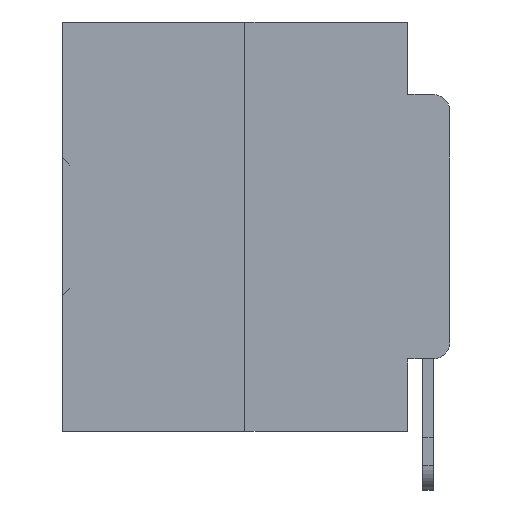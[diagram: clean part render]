
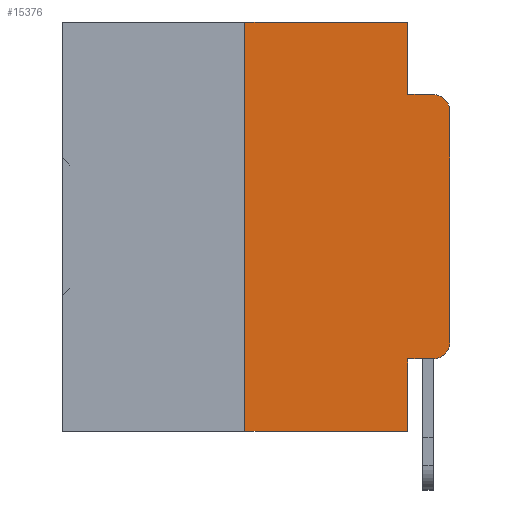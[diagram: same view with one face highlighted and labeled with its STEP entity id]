
A CAD part, left-side view. The second image highlights one B-rep face of the part: STEP entity #15376.
In plain terms, the highlighted planar face has unit normal (-1, 0, 0).
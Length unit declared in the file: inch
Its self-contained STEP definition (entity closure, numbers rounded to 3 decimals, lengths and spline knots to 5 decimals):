
#471 = CARTESIAN_POINT ( 'NONE',  ( 0., 0.02, -0.0885 ) ) ;
#874 = VECTOR ( 'NONE', #18896, 39.37008 ) ;
#1445 = VERTEX_POINT ( 'NONE', #471 ) ;
#1969 = LINE ( 'NONE', #17350, #16492 ) ;
#2561 = VECTOR ( 'NONE', #5907, 39.37008 ) ;
#3018 = DIRECTION ( 'NONE',  ( 0., 0., 1. ) ) ;
#3199 = EDGE_CURVE ( 'NONE', #34035, #13977, #10397, .T. ) ;
#3490 = LINE ( 'NONE', #34372, #25398 ) ;
#3842 = VERTEX_POINT ( 'NONE', #23069 ) ;
#4483 = EDGE_LOOP ( 'NONE', ( #11422, #12187, #13120, #13245, #14079, #14482, #14548, #14846, #14946, #15861 ) ) ;
#4899 = DIRECTION ( 'NONE',  ( -1., 0., 0. ) ) ;
#5907 = DIRECTION ( 'NONE',  ( 0., 0., -1. ) ) ;
#6653 = VERTEX_POINT ( 'NONE', #32806 ) ;
#7914 = EDGE_CURVE ( 'NONE', #28698, #6653, #32557, .T. ) ;
#8669 = PLANE ( 'NONE',  #24336 ) ;
#8960 = VECTOR ( 'NONE', #3018, 39.37008 ) ;
#9853 = CARTESIAN_POINT ( 'NONE',  ( 0., 0.051, -0.4115 ) ) ;
#10044 = EDGE_CURVE ( 'NONE', #27530, #11202, #34111, .T. ) ;
#10397 = LINE ( 'NONE', #20158, #2561 ) ;
#10764 = FACE_OUTER_BOUND ( 'NONE', #4483, .T. ) ;
#11067 = EDGE_CURVE ( 'NONE', #16762, #3842, #1969, .T. ) ;
#11202 = VERTEX_POINT ( 'NONE', #20789 ) ;
#11422 = ORIENTED_EDGE ( 'NONE', *, *, #26827, .T. ) ;
#11485 = LINE ( 'NONE', #9853, #19003 ) ;
#11572 = DIRECTION ( 'NONE',  ( 1., 0., 0. ) ) ;
#12187 = ORIENTED_EDGE ( 'NONE', *, *, #23247, .T. ) ;
#12735 = DIRECTION ( 'NONE',  ( 0., -1., 0. ) ) ;
#12960 = DIRECTION ( 'NONE',  ( 0., -1., 0. ) ) ;
#13120 = ORIENTED_EDGE ( 'NONE', *, *, #17575, .F. ) ;
#13232 = CIRCLE ( 'NONE', #33168, 0.02 ) ;
#13245 = ORIENTED_EDGE ( 'NONE', *, *, #10044, .F. ) ;
#13977 = VERTEX_POINT ( 'NONE', #35650 ) ;
#14079 = ORIENTED_EDGE ( 'NONE', *, *, #27481, .F. ) ;
#14482 = ORIENTED_EDGE ( 'NONE', *, *, #11067, .F. ) ;
#14548 = ORIENTED_EDGE ( 'NONE', *, *, #27076, .T. ) ;
#14846 = ORIENTED_EDGE ( 'NONE', *, *, #3199, .F. ) ;
#14858 = DIRECTION ( 'NONE',  ( -1., 0., 0. ) ) ;
#14946 = ORIENTED_EDGE ( 'NONE', *, *, #17477, .T. ) ;
#15376 = ADVANCED_FACE ( 'NONE', ( #10764 ), #8669, .F. ) ;
#15643 = LINE ( 'NONE', #20247, #8960 ) ;
#15861 = ORIENTED_EDGE ( 'NONE', *, *, #7914, .T. ) ;
#16492 = VECTOR ( 'NONE', #20188, 39.37008 ) ;
#16762 = VERTEX_POINT ( 'NONE', #34715 ) ;
#17074 = VECTOR ( 'NONE', #12960, 39.37008 ) ;
#17350 = CARTESIAN_POINT ( 'NONE',  ( 0., 0.25, 0. ) ) ;
#17477 = EDGE_CURVE ( 'NONE', #34035, #28698, #11485, .T. ) ;
#17575 = EDGE_CURVE ( 'NONE', #11202, #1445, #24713, .T. ) ;
#18618 = CARTESIAN_POINT ( 'NONE',  ( 0., 0.473, -0.5 ) ) ;
#18896 = DIRECTION ( 'NONE',  ( 0., -1., 0. ) ) ;
#19003 = VECTOR ( 'NONE', #12735, 39.37008 ) ;
#19226 = VECTOR ( 'NONE', #32627, 39.37008 ) ;
#20158 = CARTESIAN_POINT ( 'NONE',  ( 0., 0.051, 0. ) ) ;
#20188 = DIRECTION ( 'NONE',  ( 0., 0., 1. ) ) ;
#20247 = CARTESIAN_POINT ( 'NONE',  ( 0., 0., 0. ) ) ;
#20789 = CARTESIAN_POINT ( 'NONE',  ( 0., 0.051, -0.0885 ) ) ;
#22041 = CARTESIAN_POINT ( 'NONE',  ( 0., 0.02, -0.1085 ) ) ;
#23069 = CARTESIAN_POINT ( 'NONE',  ( 0., 0.25, 0. ) ) ;
#23247 = EDGE_CURVE ( 'NONE', #31879, #1445, #13232, .T. ) ;
#24181 = CARTESIAN_POINT ( 'NONE',  ( 0., 0.051, 0. ) ) ;
#24336 = AXIS2_PLACEMENT_3D ( 'NONE', #28466, #11572, #31287 ) ;
#24564 = LINE ( 'NONE', #18618, #17074 ) ;
#24713 = LINE ( 'NONE', #35591, #874 ) ;
#24844 = DIRECTION ( 'NONE',  ( 0., 0., -1. ) ) ;
#25398 = VECTOR ( 'NONE', #26079, 39.37008 ) ;
#26079 = DIRECTION ( 'NONE',  ( 0., -1., 0. ) ) ;
#26205 = CARTESIAN_POINT ( 'NONE',  ( 0., 0.051, 0. ) ) ;
#26827 = EDGE_CURVE ( 'NONE', #6653, #31879, #15643, .T. ) ;
#26956 = AXIS2_PLACEMENT_3D ( 'NONE', #31709, #14858, #34448 ) ;
#27076 = EDGE_CURVE ( 'NONE', #16762, #13977, #24564, .T. ) ;
#27481 = EDGE_CURVE ( 'NONE', #3842, #27530, #3490, .T. ) ;
#27530 = VERTEX_POINT ( 'NONE', #26205 ) ;
#27608 = CARTESIAN_POINT ( 'NONE',  ( 0., 0., -0.1085 ) ) ;
#27912 = CARTESIAN_POINT ( 'NONE',  ( 0., 0.02, -0.4115 ) ) ;
#28466 = CARTESIAN_POINT ( 'NONE',  ( 0., 0.473, 0. ) ) ;
#28698 = VERTEX_POINT ( 'NONE', #27912 ) ;
#30472 = CARTESIAN_POINT ( 'NONE',  ( 0., 0.051, -0.4115 ) ) ;
#31287 = DIRECTION ( 'NONE',  ( 0., 0., -1. ) ) ;
#31709 = CARTESIAN_POINT ( 'NONE',  ( 0., 0.02, -0.3915 ) ) ;
#31879 = VERTEX_POINT ( 'NONE', #27608 ) ;
#32557 = CIRCLE ( 'NONE', #26956, 0.02 ) ;
#32627 = DIRECTION ( 'NONE',  ( 0., 0., -1. ) ) ;
#32806 = CARTESIAN_POINT ( 'NONE',  ( 0., 0., -0.3915 ) ) ;
#33168 = AXIS2_PLACEMENT_3D ( 'NONE', #22041, #4899, #24844 ) ;
#34035 = VERTEX_POINT ( 'NONE', #30472 ) ;
#34111 = LINE ( 'NONE', #24181, #19226 ) ;
#34372 = CARTESIAN_POINT ( 'NONE',  ( 0., 0.473, 0. ) ) ;
#34448 = DIRECTION ( 'NONE',  ( 0., 0., -1. ) ) ;
#34715 = CARTESIAN_POINT ( 'NONE',  ( 0., 0.25, -0.5 ) ) ;
#35591 = CARTESIAN_POINT ( 'NONE',  ( 0., 0.051, -0.0885 ) ) ;
#35650 = CARTESIAN_POINT ( 'NONE',  ( 0., 0.051, -0.5 ) ) ;
